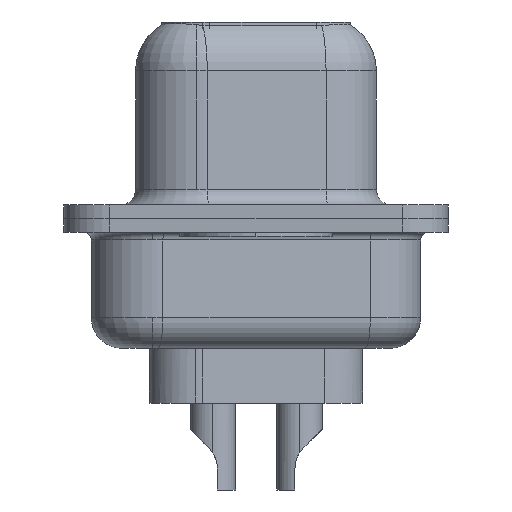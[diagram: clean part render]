
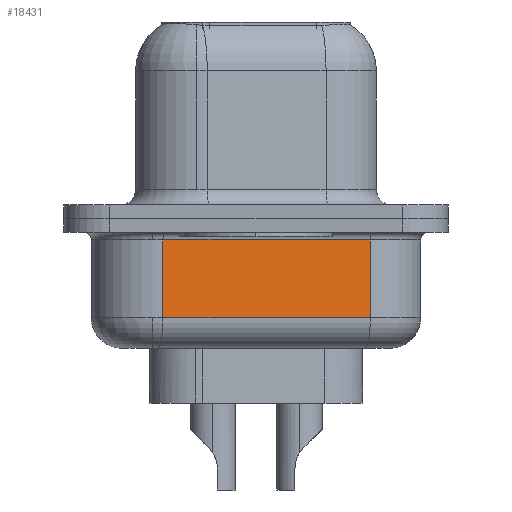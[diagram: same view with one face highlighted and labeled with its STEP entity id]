
A CAD part, left-side view. The second image highlights one B-rep face of the part: STEP entity #18431.
In plain terms, the highlighted planar face has unit normal (-0.985, -0.174, 0).
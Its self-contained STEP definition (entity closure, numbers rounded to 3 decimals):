
#275 = EDGE_CURVE ( 'NONE', #14315, #5560, #16244, .T. ) ;
#2177 = CARTESIAN_POINT ( 'NONE',  ( 2.89, 3.053, -4.25 ) ) ;
#2345 = AXIS2_PLACEMENT_3D ( 'NONE', #2177, #15460, #9515 ) ;
#2560 = DIRECTION ( 'NONE',  ( 0.174, -0.985, 0. ) ) ;
#3297 = ORIENTED_EDGE ( 'NONE', *, *, #275, .T. ) ;
#4359 = CARTESIAN_POINT ( 'NONE',  ( 2.89, 3.053, -3.25 ) ) ;
#4861 = VERTEX_POINT ( 'NONE', #11711 ) ;
#4946 = EDGE_CURVE ( 'NONE', #4861, #13852, #12556, .T. ) ;
#4949 = LINE ( 'NONE', #13952, #9438 ) ;
#5067 = CARTESIAN_POINT ( 'NONE',  ( 2.89, 3.053, -3.25 ) ) ;
#5169 = DIRECTION ( 'NONE',  ( -0.174, 0.985, 0. ) ) ;
#5179 = PLANE ( 'NONE',  #2345 ) ;
#5560 = VERTEX_POINT ( 'NONE', #8473 ) ;
#7440 = EDGE_CURVE ( 'NONE', #14315, #13852, #4949, .T. ) ;
#8473 = CARTESIAN_POINT ( 'NONE',  ( 4.089, -3.747, -3.25 ) ) ;
#8819 = EDGE_CURVE ( 'NONE', #5560, #4861, #12098, .T. ) ;
#9384 = DIRECTION ( 'NONE',  ( 0., 0., 1. ) ) ;
#9438 = VECTOR ( 'NONE', #9384, 1000. ) ;
#9483 = VECTOR ( 'NONE', #10528, 1000. ) ;
#9515 = DIRECTION ( 'NONE',  ( -0.174, 0.985, 0. ) ) ;
#10520 = ORIENTED_EDGE ( 'NONE', *, *, #7440, .F. ) ;
#10528 = DIRECTION ( 'NONE',  ( 0., 0., 1. ) ) ;
#10814 = CARTESIAN_POINT ( 'NONE',  ( 4.089, -3.747, -4.25 ) ) ;
#10927 = VECTOR ( 'NONE', #2560, 1000. ) ;
#11004 = FACE_OUTER_BOUND ( 'NONE', #11902, .T. ) ;
#11406 = CARTESIAN_POINT ( 'NONE',  ( 2.89, 3.053, -0.7 ) ) ;
#11711 = CARTESIAN_POINT ( 'NONE',  ( 4.089, -3.747, -0.7 ) ) ;
#11902 = EDGE_LOOP ( 'NONE', ( #10520, #3297, #18997, #17911 ) ) ;
#12098 = LINE ( 'NONE', #10814, #9483 ) ;
#12556 = LINE ( 'NONE', #15740, #15198 ) ;
#13852 = VERTEX_POINT ( 'NONE', #11406 ) ;
#13952 = CARTESIAN_POINT ( 'NONE',  ( 2.89, 3.053, -4.25 ) ) ;
#14315 = VERTEX_POINT ( 'NONE', #5067 ) ;
#15198 = VECTOR ( 'NONE', #5169, 1000. ) ;
#15460 = DIRECTION ( 'NONE',  ( 0.985, 0.174, 0. ) ) ;
#15740 = CARTESIAN_POINT ( 'NONE',  ( 2.89, 3.053, -0.7 ) ) ;
#16244 = LINE ( 'NONE', #4359, #10927 ) ;
#17911 = ORIENTED_EDGE ( 'NONE', *, *, #4946, .T. ) ;
#18431 = ADVANCED_FACE ( 'NONE', ( #11004 ), #5179, .F. ) ;
#18997 = ORIENTED_EDGE ( 'NONE', *, *, #8819, .T. ) ;
